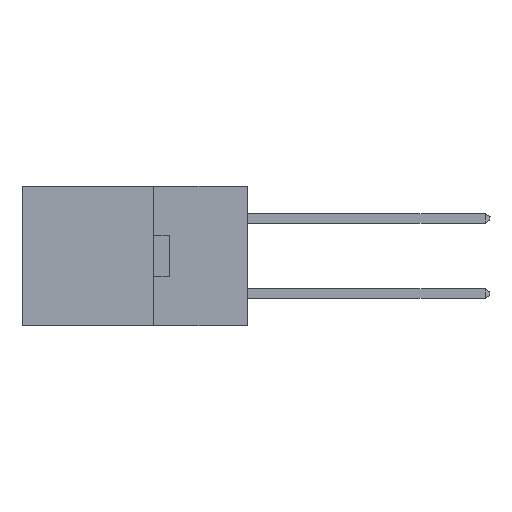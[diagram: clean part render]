
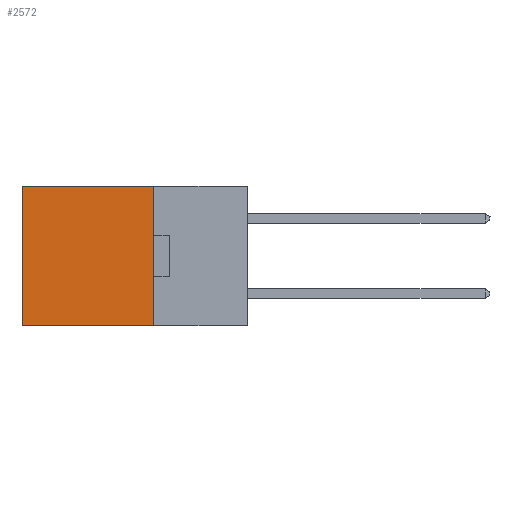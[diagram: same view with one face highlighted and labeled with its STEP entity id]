
A CAD part, left-side view. The second image highlights one B-rep face of the part: STEP entity #2572.
In plain terms, the highlighted planar face has unit normal (-1, 0, 0).
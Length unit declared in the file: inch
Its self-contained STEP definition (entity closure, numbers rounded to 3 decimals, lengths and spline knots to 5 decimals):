
#606 = VECTOR ( 'NONE', #21860, 39.37008 ) ;
#932 = LINE ( 'NONE', #24513, #19948 ) ;
#2203 = DIRECTION ( 'NONE',  ( 0., 0., -1. ) ) ;
#2572 = ADVANCED_FACE ( 'NONE', ( #23128 ), #12495, .F. ) ;
#2743 = EDGE_CURVE ( 'NONE', #27651, #25660, #932, .T. ) ;
#3996 = EDGE_CURVE ( 'NONE', #25660, #18707, #8957, .T. ) ;
#5225 = EDGE_CURVE ( 'NONE', #17875, #18707, #15160, .T. ) ;
#5301 = ORIENTED_EDGE ( 'NONE', *, *, #8944, .T. ) ;
#5590 = DIRECTION ( 'NONE',  ( 0., 1., 0. ) ) ;
#6421 = DIRECTION ( 'NONE',  ( 0., 1., 0. ) ) ;
#7388 = DIRECTION ( 'NONE',  ( 0., 0., -1. ) ) ;
#8944 = EDGE_CURVE ( 'NONE', #27651, #17875, #18402, .T. ) ;
#8957 = LINE ( 'NONE', #11337, #14446 ) ;
#9742 = CARTESIAN_POINT ( 'NONE',  ( 0.2615, 0.25, -0.37 ) ) ;
#9884 = CARTESIAN_POINT ( 'NONE',  ( 0.2615, 0.6, 0. ) ) ;
#10208 = ORIENTED_EDGE ( 'NONE', *, *, #5225, .T. ) ;
#11337 = CARTESIAN_POINT ( 'NONE',  ( 0.2615, 0.25, -0.37 ) ) ;
#12248 = VECTOR ( 'NONE', #5590, 39.37008 ) ;
#12495 = PLANE ( 'NONE',  #13896 ) ;
#13896 = AXIS2_PLACEMENT_3D ( 'NONE', #26057, #21706, #2203 ) ;
#14446 = VECTOR ( 'NONE', #6421, 39.37008 ) ;
#15160 = LINE ( 'NONE', #25793, #606 ) ;
#17875 = VERTEX_POINT ( 'NONE', #9884 ) ;
#18402 = LINE ( 'NONE', #22998, #12248 ) ;
#18707 = VERTEX_POINT ( 'NONE', #24410 ) ;
#19948 = VECTOR ( 'NONE', #7388, 39.37008 ) ;
#21108 = ORIENTED_EDGE ( 'NONE', *, *, #3996, .F. ) ;
#21159 = ORIENTED_EDGE ( 'NONE', *, *, #2743, .F. ) ;
#21706 = DIRECTION ( 'NONE',  ( 1., 0., 0. ) ) ;
#21860 = DIRECTION ( 'NONE',  ( 0., 0., -1. ) ) ;
#22998 = CARTESIAN_POINT ( 'NONE',  ( 0.2615, 0.25, 0. ) ) ;
#23128 = FACE_OUTER_BOUND ( 'NONE', #25609, .T. ) ;
#24410 = CARTESIAN_POINT ( 'NONE',  ( 0.2615, 0.6, -0.37 ) ) ;
#24513 = CARTESIAN_POINT ( 'NONE',  ( 0.2615, 0.25, -0.37 ) ) ;
#25268 = CARTESIAN_POINT ( 'NONE',  ( 0.2615, 0.25, 0. ) ) ;
#25609 = EDGE_LOOP ( 'NONE', ( #10208, #21108, #21159, #5301 ) ) ;
#25660 = VERTEX_POINT ( 'NONE', #9742 ) ;
#25793 = CARTESIAN_POINT ( 'NONE',  ( 0.2615, 0.6, -0.37 ) ) ;
#26057 = CARTESIAN_POINT ( 'NONE',  ( 0.2615, 0.25, -0.37 ) ) ;
#27651 = VERTEX_POINT ( 'NONE', #25268 ) ;
